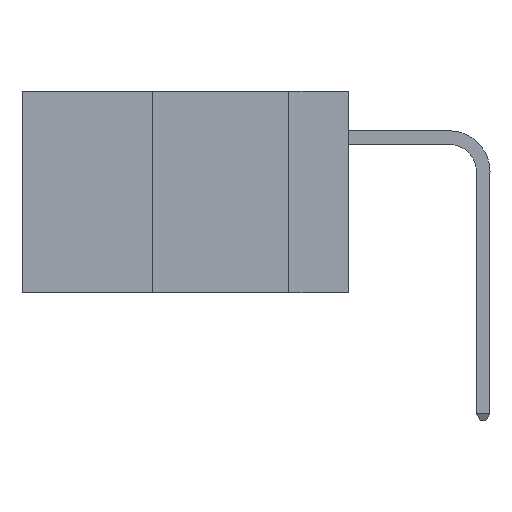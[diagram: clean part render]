
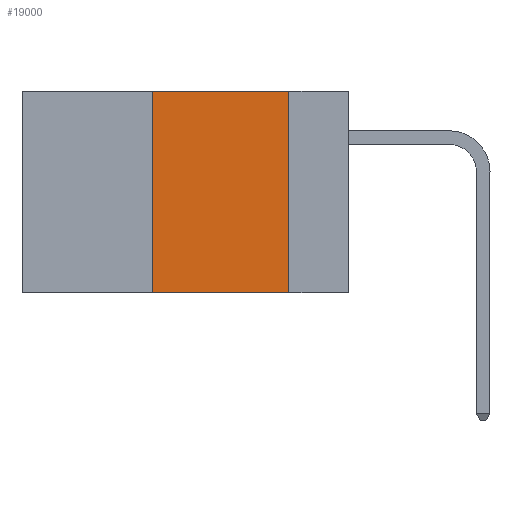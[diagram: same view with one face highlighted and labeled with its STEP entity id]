
A CAD part, left-side view. The second image highlights one B-rep face of the part: STEP entity #19000.
In plain terms, the highlighted planar face has unit normal (-1, 0, 0).
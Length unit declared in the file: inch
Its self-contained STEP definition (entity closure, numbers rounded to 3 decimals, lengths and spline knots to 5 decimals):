
#181 = LINE ( 'NONE', #10844, #21051 ) ;
#473 = VERTEX_POINT ( 'NONE', #11710 ) ;
#559 = CARTESIAN_POINT ( 'NONE',  ( 0., 0.11, 0. ) ) ;
#2066 = VECTOR ( 'NONE', #17446, 39.37008 ) ;
#2204 = CARTESIAN_POINT ( 'NONE',  ( 0., 0.6, 0. ) ) ;
#2264 = CARTESIAN_POINT ( 'NONE',  ( 0., 0.6, 0. ) ) ;
#3469 = ORIENTED_EDGE ( 'NONE', *, *, #13624, .T. ) ;
#3595 = VERTEX_POINT ( 'NONE', #8904 ) ;
#4838 = EDGE_CURVE ( 'NONE', #17656, #5644, #181, .T. ) ;
#5202 = CARTESIAN_POINT ( 'NONE',  ( 0., 0.36, -0.37 ) ) ;
#5644 = VERTEX_POINT ( 'NONE', #13228 ) ;
#5768 = CARTESIAN_POINT ( 'NONE',  ( 0., 0.6, -0.37 ) ) ;
#6183 = ORIENTED_EDGE ( 'NONE', *, *, #8213, .F. ) ;
#8213 = EDGE_CURVE ( 'NONE', #5644, #473, #9118, .T. ) ;
#8601 = AXIS2_PLACEMENT_3D ( 'NONE', #2264, #20810, #10796 ) ;
#8904 = CARTESIAN_POINT ( 'NONE',  ( 0., 0.11, -0.37 ) ) ;
#9118 = LINE ( 'NONE', #2204, #18037 ) ;
#10796 = DIRECTION ( 'NONE',  ( 0., 0., -1. ) ) ;
#10820 = EDGE_LOOP ( 'NONE', ( #18568, #6183, #15864, #3469 ) ) ;
#10844 = CARTESIAN_POINT ( 'NONE',  ( 0., 0.36, 0. ) ) ;
#11095 = LINE ( 'NONE', #559, #2066 ) ;
#11710 = CARTESIAN_POINT ( 'NONE',  ( 0., 0.11, 0. ) ) ;
#12580 = DIRECTION ( 'NONE',  ( 0., -1., 0. ) ) ;
#13228 = CARTESIAN_POINT ( 'NONE',  ( 0., 0.36, 0. ) ) ;
#13624 = EDGE_CURVE ( 'NONE', #17656, #3595, #18192, .T. ) ;
#14022 = DIRECTION ( 'NONE',  ( 0., -1., 0. ) ) ;
#14198 = EDGE_CURVE ( 'NONE', #473, #3595, #11095, .T. ) ;
#14720 = FACE_OUTER_BOUND ( 'NONE', #10820, .T. ) ;
#15864 = ORIENTED_EDGE ( 'NONE', *, *, #4838, .F. ) ;
#15900 = DIRECTION ( 'NONE',  ( 0., 0., 1. ) ) ;
#17446 = DIRECTION ( 'NONE',  ( 0., 0., -1. ) ) ;
#17656 = VERTEX_POINT ( 'NONE', #5202 ) ;
#17680 = VECTOR ( 'NONE', #12580, 39.37008 ) ;
#18037 = VECTOR ( 'NONE', #14022, 39.37008 ) ;
#18192 = LINE ( 'NONE', #5768, #17680 ) ;
#18568 = ORIENTED_EDGE ( 'NONE', *, *, #14198, .F. ) ;
#19000 = ADVANCED_FACE ( 'NONE', ( #14720 ), #19146, .F. ) ;
#19146 = PLANE ( 'NONE',  #8601 ) ;
#20810 = DIRECTION ( 'NONE',  ( 1., 0., 0. ) ) ;
#21051 = VECTOR ( 'NONE', #15900, 39.37008 ) ;
